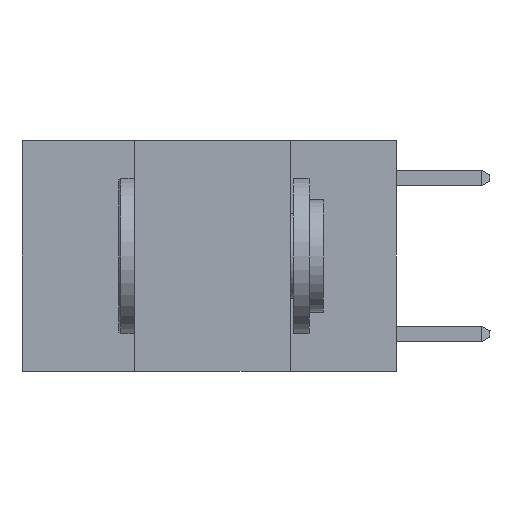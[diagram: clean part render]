
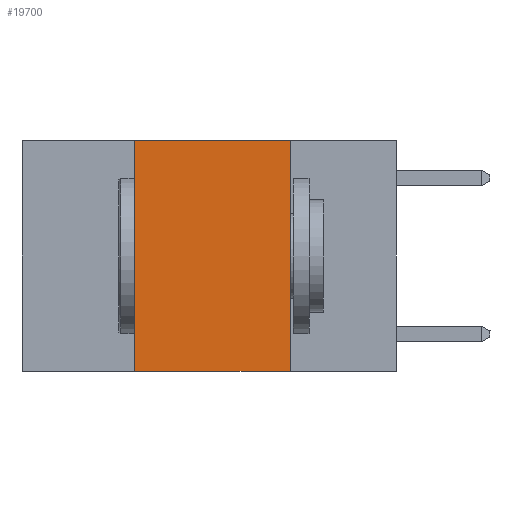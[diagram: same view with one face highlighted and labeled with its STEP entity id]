
A CAD part, left-side view. The second image highlights one B-rep face of the part: STEP entity #19700.
In plain terms, the highlighted planar face has unit normal (-1, 0, 0).
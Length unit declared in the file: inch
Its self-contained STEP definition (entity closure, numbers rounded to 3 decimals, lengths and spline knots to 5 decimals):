
#916 = VECTOR ( 'NONE', #18768, 39.37008 ) ;
#1513 = LINE ( 'NONE', #10628, #20680 ) ;
#1670 = LINE ( 'NONE', #9187, #916 ) ;
#3515 = CARTESIAN_POINT ( 'NONE',  ( 0., 0.42, -0.37 ) ) ;
#3639 = EDGE_CURVE ( 'NONE', #4251, #10473, #1670, .T. ) ;
#3965 = VERTEX_POINT ( 'NONE', #3515 ) ;
#3966 = DIRECTION ( 'NONE',  ( 0., -1., 0. ) ) ;
#4229 = ORIENTED_EDGE ( 'NONE', *, *, #7927, .F. ) ;
#4251 = VERTEX_POINT ( 'NONE', #18938 ) ;
#6288 = VECTOR ( 'NONE', #29358, 39.37008 ) ;
#7016 = EDGE_LOOP ( 'NONE', ( #17871, #17237, #4229, #24270 ) ) ;
#7927 = EDGE_CURVE ( 'NONE', #3965, #4251, #1513, .T. ) ;
#8218 = FACE_OUTER_BOUND ( 'NONE', #7016, .T. ) ;
#9187 = CARTESIAN_POINT ( 'NONE',  ( 0., 0.6, 0. ) ) ;
#10088 = CARTESIAN_POINT ( 'NONE',  ( 0., 0.6, 0. ) ) ;
#10473 = VERTEX_POINT ( 'NONE', #19382 ) ;
#10628 = CARTESIAN_POINT ( 'NONE',  ( 0., 0.42, 0. ) ) ;
#10930 = CARTESIAN_POINT ( 'NONE',  ( 0., 0.17, 0. ) ) ;
#13488 = LINE ( 'NONE', #10930, #6288 ) ;
#14916 = DIRECTION ( 'NONE',  ( 0., 0., -1. ) ) ;
#15673 = EDGE_CURVE ( 'NONE', #3965, #21392, #22941, .T. ) ;
#15948 = AXIS2_PLACEMENT_3D ( 'NONE', #10088, #28508, #14916 ) ;
#17237 = ORIENTED_EDGE ( 'NONE', *, *, #3639, .F. ) ;
#17602 = CARTESIAN_POINT ( 'NONE',  ( 0., 0.17, -0.37 ) ) ;
#17871 = ORIENTED_EDGE ( 'NONE', *, *, #19987, .F. ) ;
#18768 = DIRECTION ( 'NONE',  ( 0., -1., 0. ) ) ;
#18938 = CARTESIAN_POINT ( 'NONE',  ( 0., 0.42, 0. ) ) ;
#19382 = CARTESIAN_POINT ( 'NONE',  ( 0., 0.17, 0. ) ) ;
#19700 = ADVANCED_FACE ( 'NONE', ( #8218 ), #24078, .F. ) ;
#19987 = EDGE_CURVE ( 'NONE', #10473, #21392, #13488, .T. ) ;
#20680 = VECTOR ( 'NONE', #24574, 39.37008 ) ;
#21392 = VERTEX_POINT ( 'NONE', #17602 ) ;
#22941 = LINE ( 'NONE', #29549, #28161 ) ;
#24078 = PLANE ( 'NONE',  #15948 ) ;
#24270 = ORIENTED_EDGE ( 'NONE', *, *, #15673, .T. ) ;
#24574 = DIRECTION ( 'NONE',  ( 0., 0., 1. ) ) ;
#28161 = VECTOR ( 'NONE', #3966, 39.37008 ) ;
#28508 = DIRECTION ( 'NONE',  ( 1., 0., 0. ) ) ;
#29358 = DIRECTION ( 'NONE',  ( 0., 0., -1. ) ) ;
#29549 = CARTESIAN_POINT ( 'NONE',  ( 0., 0.6, -0.37 ) ) ;
